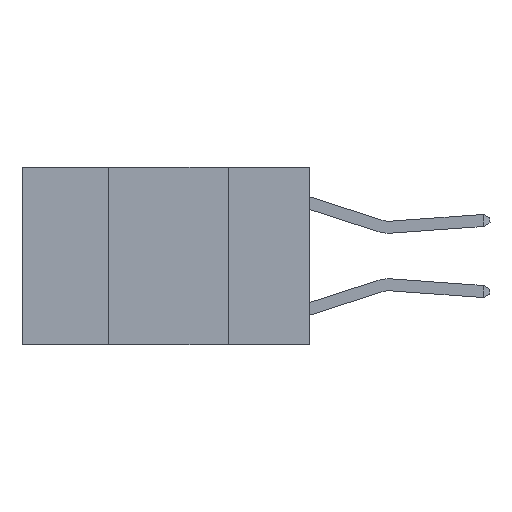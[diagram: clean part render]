
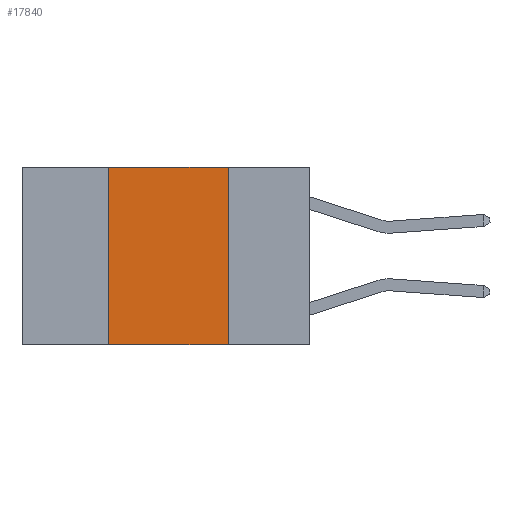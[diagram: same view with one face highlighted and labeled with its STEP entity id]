
A CAD part, left-side view. The second image highlights one B-rep face of the part: STEP entity #17840.
In plain terms, the highlighted planar face has unit normal (-1, 0, 0).
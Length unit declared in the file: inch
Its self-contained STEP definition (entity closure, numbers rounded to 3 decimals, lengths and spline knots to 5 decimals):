
#108 = ORIENTED_EDGE ( 'NONE', *, *, #12934, .F. ) ;
#236 = EDGE_CURVE ( 'NONE', #16551, #19028, #17674, .T. ) ;
#2573 = LINE ( 'NONE', #16608, #20509 ) ;
#4186 = CARTESIAN_POINT ( 'NONE',  ( 0., 0.6, 0. ) ) ;
#4258 = VECTOR ( 'NONE', #4852, 39.37008 ) ;
#4601 = DIRECTION ( 'NONE',  ( 0., -1., 0. ) ) ;
#4852 = DIRECTION ( 'NONE',  ( 0., 0., 1. ) ) ;
#5115 = LINE ( 'NONE', #10800, #5682 ) ;
#5503 = VERTEX_POINT ( 'NONE', #5655 ) ;
#5655 = CARTESIAN_POINT ( 'NONE',  ( 0., 0.42, -0.37 ) ) ;
#5682 = VECTOR ( 'NONE', #7404, 39.37008 ) ;
#5981 = DIRECTION ( 'NONE',  ( 0., 0., -1. ) ) ;
#7404 = DIRECTION ( 'NONE',  ( 0., -1., 0. ) ) ;
#8510 = VECTOR ( 'NONE', #9784, 39.37008 ) ;
#9784 = DIRECTION ( 'NONE',  ( 0., 0., -1. ) ) ;
#9952 = ORIENTED_EDGE ( 'NONE', *, *, #10353, .T. ) ;
#10353 = EDGE_CURVE ( 'NONE', #5503, #19028, #5115, .T. ) ;
#10800 = CARTESIAN_POINT ( 'NONE',  ( 0., 0.6, -0.37 ) ) ;
#11088 = PLANE ( 'NONE',  #20369 ) ;
#12629 = CARTESIAN_POINT ( 'NONE',  ( 0., 0.17, -0.37 ) ) ;
#12813 = FACE_OUTER_BOUND ( 'NONE', #21182, .T. ) ;
#12911 = ORIENTED_EDGE ( 'NONE', *, *, #13444, .F. ) ;
#12934 = EDGE_CURVE ( 'NONE', #5503, #17667, #13447, .T. ) ;
#13444 = EDGE_CURVE ( 'NONE', #17667, #16551, #2573, .T. ) ;
#13447 = LINE ( 'NONE', #16942, #4258 ) ;
#15905 = CARTESIAN_POINT ( 'NONE',  ( 0., 0.42, 0. ) ) ;
#16276 = DIRECTION ( 'NONE',  ( 1., 0., 0. ) ) ;
#16551 = VERTEX_POINT ( 'NONE', #17400 ) ;
#16608 = CARTESIAN_POINT ( 'NONE',  ( 0., 0.6, 0. ) ) ;
#16942 = CARTESIAN_POINT ( 'NONE',  ( 0., 0.42, 0. ) ) ;
#17400 = CARTESIAN_POINT ( 'NONE',  ( 0., 0.17, 0. ) ) ;
#17667 = VERTEX_POINT ( 'NONE', #15905 ) ;
#17674 = LINE ( 'NONE', #20011, #8510 ) ;
#17840 = ADVANCED_FACE ( 'NONE', ( #12813 ), #11088, .F. ) ;
#19028 = VERTEX_POINT ( 'NONE', #12629 ) ;
#20011 = CARTESIAN_POINT ( 'NONE',  ( 0., 0.17, 0. ) ) ;
#20369 = AXIS2_PLACEMENT_3D ( 'NONE', #4186, #16276, #5981 ) ;
#20509 = VECTOR ( 'NONE', #4601, 39.37008 ) ;
#21182 = EDGE_LOOP ( 'NONE', ( #21589, #12911, #108, #9952 ) ) ;
#21589 = ORIENTED_EDGE ( 'NONE', *, *, #236, .F. ) ;
